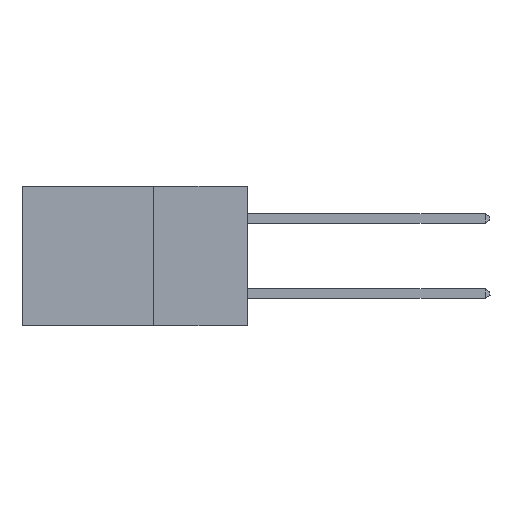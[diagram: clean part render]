
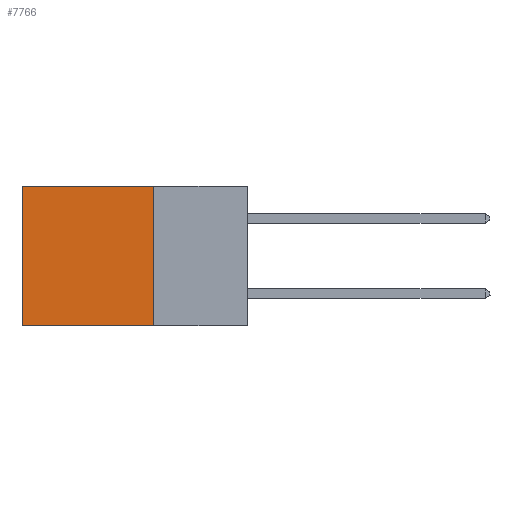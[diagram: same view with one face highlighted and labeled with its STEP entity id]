
A CAD part, left-side view. The second image highlights one B-rep face of the part: STEP entity #7766.
In plain terms, the highlighted planar face has unit normal (-1, 0, 0).
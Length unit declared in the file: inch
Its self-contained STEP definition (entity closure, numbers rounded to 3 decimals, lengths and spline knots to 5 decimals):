
#1460 = VECTOR ( 'NONE', #9797, 39.37008 ) ;
#1791 = DIRECTION ( 'NONE',  ( 0., 0., -1. ) ) ;
#2351 = DIRECTION ( 'NONE',  ( 0., 0., -1. ) ) ;
#2698 = CARTESIAN_POINT ( 'NONE',  ( 0.298, 0.25, 0. ) ) ;
#2780 = VERTEX_POINT ( 'NONE', #23236 ) ;
#4164 = EDGE_CURVE ( 'NONE', #6252, #24747, #15479, .T. ) ;
#5056 = ORIENTED_EDGE ( 'NONE', *, *, #19552, .T. ) ;
#5118 = CARTESIAN_POINT ( 'NONE',  ( 0.298, 0.25, -0.37 ) ) ;
#6252 = VERTEX_POINT ( 'NONE', #6465 ) ;
#6465 = CARTESIAN_POINT ( 'NONE',  ( 0.298, 0.6, 0. ) ) ;
#6577 = LINE ( 'NONE', #12475, #26655 ) ;
#6696 = CARTESIAN_POINT ( 'NONE',  ( 0.298, 0.25, 0. ) ) ;
#7766 = ADVANCED_FACE ( 'NONE', ( #16790 ), #28639, .F. ) ;
#7948 = VECTOR ( 'NONE', #20097, 39.37008 ) ;
#8402 = EDGE_CURVE ( 'NONE', #2780, #24747, #19887, .T. ) ;
#8990 = DIRECTION ( 'NONE',  ( 1., 0., 0. ) ) ;
#9607 = VECTOR ( 'NONE', #1791, 39.37008 ) ;
#9797 = DIRECTION ( 'NONE',  ( 0., 1., 0. ) ) ;
#9979 = ORIENTED_EDGE ( 'NONE', *, *, #24945, .F. ) ;
#10029 = LINE ( 'NONE', #2698, #7948 ) ;
#11340 = EDGE_LOOP ( 'NONE', ( #18226, #23104, #9979, #5056 ) ) ;
#12475 = CARTESIAN_POINT ( 'NONE',  ( 0.298, 0.25, 0. ) ) ;
#15459 = CARTESIAN_POINT ( 'NONE',  ( 0.298, 0.25, 0. ) ) ;
#15479 = LINE ( 'NONE', #25442, #9607 ) ;
#16395 = AXIS2_PLACEMENT_3D ( 'NONE', #15459, #8990, #2351 ) ;
#16790 = FACE_OUTER_BOUND ( 'NONE', #11340, .T. ) ;
#18226 = ORIENTED_EDGE ( 'NONE', *, *, #4164, .T. ) ;
#18786 = DIRECTION ( 'NONE',  ( 0., 0., -1. ) ) ;
#19552 = EDGE_CURVE ( 'NONE', #20004, #6252, #10029, .T. ) ;
#19887 = LINE ( 'NONE', #5118, #1460 ) ;
#20004 = VERTEX_POINT ( 'NONE', #6696 ) ;
#20097 = DIRECTION ( 'NONE',  ( 0., 1., 0. ) ) ;
#20226 = CARTESIAN_POINT ( 'NONE',  ( 0.298, 0.6, -0.37 ) ) ;
#23104 = ORIENTED_EDGE ( 'NONE', *, *, #8402, .F. ) ;
#23236 = CARTESIAN_POINT ( 'NONE',  ( 0.298, 0.25, -0.37 ) ) ;
#24747 = VERTEX_POINT ( 'NONE', #20226 ) ;
#24945 = EDGE_CURVE ( 'NONE', #20004, #2780, #6577, .T. ) ;
#25442 = CARTESIAN_POINT ( 'NONE',  ( 0.298, 0.6, 0. ) ) ;
#26655 = VECTOR ( 'NONE', #18786, 39.37008 ) ;
#28639 = PLANE ( 'NONE',  #16395 ) ;
